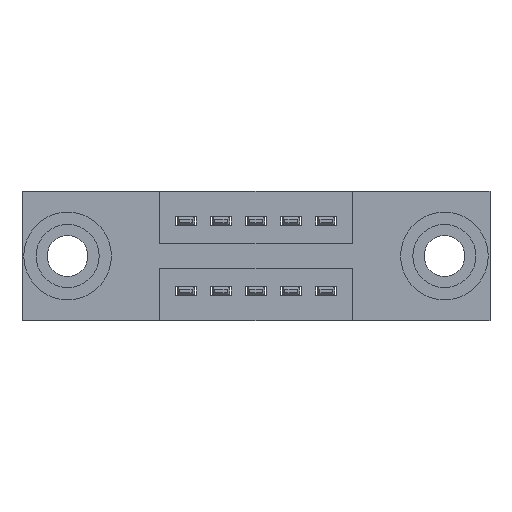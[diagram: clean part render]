
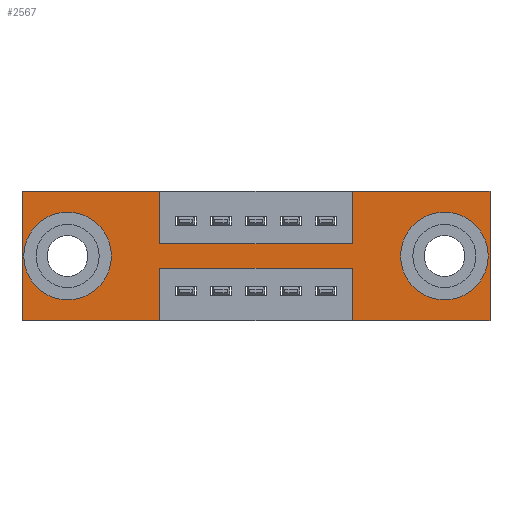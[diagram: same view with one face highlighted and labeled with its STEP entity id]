
A CAD part, front view. The second image highlights one B-rep face of the part: STEP entity #2567.
In plain terms, the highlighted planar face has unit normal (0, -1, 0).
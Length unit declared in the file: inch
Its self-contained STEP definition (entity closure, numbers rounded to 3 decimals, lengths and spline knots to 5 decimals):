
#65 = VECTOR ( 'NONE', #1583, 39.37008 ) ;
#145 = VERTEX_POINT ( 'NONE', #3130 ) ;
#159 = EDGE_CURVE ( 'NONE', #6426, #145, #5994, .T. ) ;
#169 = LINE ( 'NONE', #8756, #5517 ) ;
#308 = VECTOR ( 'NONE', #7540, 39.37008 ) ;
#326 = CIRCLE ( 'NONE', #2110, 0.078 ) ;
#493 = CARTESIAN_POINT ( 'NONE',  ( 0.13, 0., -0.185 ) ) ;
#517 = ORIENTED_EDGE ( 'NONE', *, *, #1044, .T. ) ;
#582 = VERTEX_POINT ( 'NONE', #8790 ) ;
#614 = VERTEX_POINT ( 'NONE', #8813 ) ;
#621 = CARTESIAN_POINT ( 'NONE',  ( 0., 0., 0. ) ) ;
#690 = EDGE_CURVE ( 'NONE', #4701, #8867, #5312, .T. ) ;
#831 = CIRCLE ( 'NONE', #5506, 0.078 ) ;
#846 = ORIENTED_EDGE ( 'NONE', *, *, #1298, .F. ) ;
#887 = LINE ( 'NONE', #6452, #8388 ) ;
#968 = DIRECTION ( 'NONE',  ( 0., 1., 0. ) ) ;
#993 = DIRECTION ( 'NONE',  ( 1., 0., 0. ) ) ;
#1011 = VECTOR ( 'NONE', #6315, 39.37008 ) ;
#1013 = VERTEX_POINT ( 'NONE', #5634 ) ;
#1044 = EDGE_CURVE ( 'NONE', #614, #2794, #8383, .T. ) ;
#1071 = FACE_OUTER_BOUND ( 'NONE', #4939, .T. ) ;
#1221 = DIRECTION ( 'NONE',  ( 0., 0., 1. ) ) ;
#1295 = FACE_BOUND ( 'NONE', #5042, .T. ) ;
#1298 = EDGE_CURVE ( 'NONE', #582, #4701, #4637, .T. ) ;
#1324 = ORIENTED_EDGE ( 'NONE', *, *, #6569, .F. ) ;
#1416 = LINE ( 'NONE', #621, #1629 ) ;
#1502 = ORIENTED_EDGE ( 'NONE', *, *, #159, .T. ) ;
#1526 = DIRECTION ( 'NONE',  ( -1., 0., 0. ) ) ;
#1583 = DIRECTION ( 'NONE',  ( 0., 0., 1. ) ) ;
#1629 = VECTOR ( 'NONE', #4970, 39.37008 ) ;
#1725 = VERTEX_POINT ( 'NONE', #5504 ) ;
#1810 = ORIENTED_EDGE ( 'NONE', *, *, #8051, .T. ) ;
#1835 = CARTESIAN_POINT ( 'NONE',  ( 0.9425, 0., -0.15 ) ) ;
#1865 = EDGE_CURVE ( 'NONE', #8937, #7951, #1416, .T. ) ;
#1997 = CARTESIAN_POINT ( 'NONE',  ( 0., 0., -0.37 ) ) ;
#2010 = LINE ( 'NONE', #5927, #65 ) ;
#2057 = DIRECTION ( 'NONE',  ( 0., 1., 0. ) ) ;
#2110 = AXIS2_PLACEMENT_3D ( 'NONE', #493, #5560, #1221 ) ;
#2131 = ORIENTED_EDGE ( 'NONE', *, *, #690, .F. ) ;
#2348 = VECTOR ( 'NONE', #9267, 39.37008 ) ;
#2433 = VECTOR ( 'NONE', #6802, 39.37008 ) ;
#2567 = ADVANCED_FACE ( 'NONE', ( #2995, #1295, #1071 ), #4890, .T. ) ;
#2593 = EDGE_CURVE ( 'NONE', #145, #6426, #831, .T. ) ;
#2659 = ORIENTED_EDGE ( 'NONE', *, *, #6539, .F. ) ;
#2662 = VERTEX_POINT ( 'NONE', #5108 ) ;
#2727 = ORIENTED_EDGE ( 'NONE', *, *, #2593, .T. ) ;
#2742 = DIRECTION ( 'NONE',  ( 0., 0., -1. ) ) ;
#2779 = ORIENTED_EDGE ( 'NONE', *, *, #7337, .F. ) ;
#2794 = VERTEX_POINT ( 'NONE', #5947 ) ;
#2995 = FACE_BOUND ( 'NONE', #8397, .T. ) ;
#3130 = CARTESIAN_POINT ( 'NONE',  ( 1.205, 0., -0.107 ) ) ;
#3412 = VECTOR ( 'NONE', #4586, 39.37008 ) ;
#3442 = EDGE_CURVE ( 'NONE', #6153, #1013, #169, .T. ) ;
#3975 = ORIENTED_EDGE ( 'NONE', *, *, #4033, .F. ) ;
#3981 = DIRECTION ( 'NONE',  ( -1., 0., 0. ) ) ;
#4033 = EDGE_CURVE ( 'NONE', #6530, #6298, #6295, .T. ) ;
#4217 = DIRECTION ( 'NONE',  ( 0., 0., 1. ) ) ;
#4254 = DIRECTION ( 'NONE',  ( 0., 1., 0. ) ) ;
#4423 = VECTOR ( 'NONE', #4217, 39.37008 ) ;
#4586 = DIRECTION ( 'NONE',  ( 0., 0., -1. ) ) ;
#4625 = CARTESIAN_POINT ( 'NONE',  ( 0.3925, 0., -0.15 ) ) ;
#4637 = LINE ( 'NONE', #9030, #7233 ) ;
#4671 = CARTESIAN_POINT ( 'NONE',  ( 0., 0., -0.37 ) ) ;
#4701 = VERTEX_POINT ( 'NONE', #7519 ) ;
#4715 = CARTESIAN_POINT ( 'NONE',  ( 0.3925, 0., 0. ) ) ;
#4749 = LINE ( 'NONE', #4625, #8369 ) ;
#4834 = ORIENTED_EDGE ( 'NONE', *, *, #7702, .F. ) ;
#4890 = PLANE ( 'NONE',  #5021 ) ;
#4939 = EDGE_LOOP ( 'NONE', ( #2131, #846, #1324, #8876, #2659, #3975, #7909, #4834, #4950, #6850, #2779, #5372 ) ) ;
#4950 = ORIENTED_EDGE ( 'NONE', *, *, #8901, .F. ) ;
#4952 = CARTESIAN_POINT ( 'NONE',  ( 0., 0., 0. ) ) ;
#4970 = DIRECTION ( 'NONE',  ( 1., 0., 0. ) ) ;
#5021 = AXIS2_PLACEMENT_3D ( 'NONE', #1997, #7067, #2742 ) ;
#5042 = EDGE_LOOP ( 'NONE', ( #517, #1810 ) ) ;
#5108 = CARTESIAN_POINT ( 'NONE',  ( 0., 0., -0.37 ) ) ;
#5293 = CARTESIAN_POINT ( 'NONE',  ( 1.335, 0., 0. ) ) ;
#5301 = CARTESIAN_POINT ( 'NONE',  ( 1.205, 0., -0.185 ) ) ;
#5312 = LINE ( 'NONE', #8902, #3412 ) ;
#5372 = ORIENTED_EDGE ( 'NONE', *, *, #7072, .F. ) ;
#5504 = CARTESIAN_POINT ( 'NONE',  ( 0.3925, 0., -0.15 ) ) ;
#5506 = AXIS2_PLACEMENT_3D ( 'NONE', #6399, #2057, #7133 ) ;
#5517 = VECTOR ( 'NONE', #1526, 39.37008 ) ;
#5560 = DIRECTION ( 'NONE',  ( 0., 1., 0. ) ) ;
#5634 = CARTESIAN_POINT ( 'NONE',  ( 0.9425, 0., -0.37 ) ) ;
#5927 = CARTESIAN_POINT ( 'NONE',  ( 0.9425, 0., 0. ) ) ;
#5947 = CARTESIAN_POINT ( 'NONE',  ( 0.13, 0., -0.263 ) ) ;
#5968 = LINE ( 'NONE', #4952, #2348 ) ;
#5994 = CIRCLE ( 'NONE', #7185, 0.078 ) ;
#6027 = DIRECTION ( 'NONE',  ( 0., 0., -1. ) ) ;
#6065 = CARTESIAN_POINT ( 'NONE',  ( 0., 0., 0. ) ) ;
#6153 = VERTEX_POINT ( 'NONE', #8374 ) ;
#6192 = CARTESIAN_POINT ( 'NONE',  ( 1.205, 0., -0.263 ) ) ;
#6295 = LINE ( 'NONE', #6065, #2433 ) ;
#6298 = VERTEX_POINT ( 'NONE', #5293 ) ;
#6315 = DIRECTION ( 'NONE',  ( 0., 0., -1. ) ) ;
#6342 = LINE ( 'NONE', #9257, #4423 ) ;
#6399 = CARTESIAN_POINT ( 'NONE',  ( 1.205, 0., -0.185 ) ) ;
#6426 = VERTEX_POINT ( 'NONE', #6192 ) ;
#6452 = CARTESIAN_POINT ( 'NONE',  ( 0.3925, 0., 0. ) ) ;
#6522 = CARTESIAN_POINT ( 'NONE',  ( 0., 0., 0. ) ) ;
#6530 = VERTEX_POINT ( 'NONE', #7755 ) ;
#6539 = EDGE_CURVE ( 'NONE', #6298, #6153, #6785, .T. ) ;
#6569 = EDGE_CURVE ( 'NONE', #1013, #582, #6342, .T. ) ;
#6785 = LINE ( 'NONE', #8478, #1011 ) ;
#6802 = DIRECTION ( 'NONE',  ( 1., 0., 0. ) ) ;
#6850 = ORIENTED_EDGE ( 'NONE', *, *, #1865, .F. ) ;
#7067 = DIRECTION ( 'NONE',  ( 0., -1., 0. ) ) ;
#7072 = EDGE_CURVE ( 'NONE', #8867, #2662, #8034, .T. ) ;
#7133 = DIRECTION ( 'NONE',  ( 0., 0., -1. ) ) ;
#7134 = AXIS2_PLACEMENT_3D ( 'NONE', #8581, #4254, #9296 ) ;
#7185 = AXIS2_PLACEMENT_3D ( 'NONE', #5301, #968, #6027 ) ;
#7233 = VECTOR ( 'NONE', #3981, 39.37008 ) ;
#7337 = EDGE_CURVE ( 'NONE', #2662, #8937, #5968, .T. ) ;
#7519 = CARTESIAN_POINT ( 'NONE',  ( 0.3925, 0., -0.22 ) ) ;
#7540 = DIRECTION ( 'NONE',  ( -1., 0., 0. ) ) ;
#7571 = EDGE_CURVE ( 'NONE', #8010, #6530, #2010, .T. ) ;
#7702 = EDGE_CURVE ( 'NONE', #1725, #8010, #4749, .T. ) ;
#7755 = CARTESIAN_POINT ( 'NONE',  ( 0.9425, 0., 0. ) ) ;
#7909 = ORIENTED_EDGE ( 'NONE', *, *, #7571, .F. ) ;
#7916 = DIRECTION ( 'NONE',  ( 0., 0., -1. ) ) ;
#7951 = VERTEX_POINT ( 'NONE', #4715 ) ;
#8010 = VERTEX_POINT ( 'NONE', #1835 ) ;
#8034 = LINE ( 'NONE', #4671, #308 ) ;
#8051 = EDGE_CURVE ( 'NONE', #2794, #614, #326, .T. ) ;
#8369 = VECTOR ( 'NONE', #993, 39.37008 ) ;
#8374 = CARTESIAN_POINT ( 'NONE',  ( 1.335, 0., -0.37 ) ) ;
#8383 = CIRCLE ( 'NONE', #7134, 0.078 ) ;
#8388 = VECTOR ( 'NONE', #7916, 39.37008 ) ;
#8397 = EDGE_LOOP ( 'NONE', ( #2727, #1502 ) ) ;
#8478 = CARTESIAN_POINT ( 'NONE',  ( 1.335, 0., 0. ) ) ;
#8581 = CARTESIAN_POINT ( 'NONE',  ( 0.13, 0., -0.185 ) ) ;
#8613 = CARTESIAN_POINT ( 'NONE',  ( 0.3925, 0., -0.37 ) ) ;
#8756 = CARTESIAN_POINT ( 'NONE',  ( 0., 0., -0.37 ) ) ;
#8790 = CARTESIAN_POINT ( 'NONE',  ( 0.9425, 0., -0.22 ) ) ;
#8813 = CARTESIAN_POINT ( 'NONE',  ( 0.13, 0., -0.107 ) ) ;
#8867 = VERTEX_POINT ( 'NONE', #8613 ) ;
#8876 = ORIENTED_EDGE ( 'NONE', *, *, #3442, .F. ) ;
#8901 = EDGE_CURVE ( 'NONE', #7951, #1725, #887, .T. ) ;
#8902 = CARTESIAN_POINT ( 'NONE',  ( 0.3925, 0., -0.37 ) ) ;
#8937 = VERTEX_POINT ( 'NONE', #6522 ) ;
#9030 = CARTESIAN_POINT ( 'NONE',  ( 0.3925, 0., -0.22 ) ) ;
#9257 = CARTESIAN_POINT ( 'NONE',  ( 0.9425, 0., -0.37 ) ) ;
#9267 = DIRECTION ( 'NONE',  ( 0., 0., 1. ) ) ;
#9296 = DIRECTION ( 'NONE',  ( 0., 0., 1. ) ) ;
